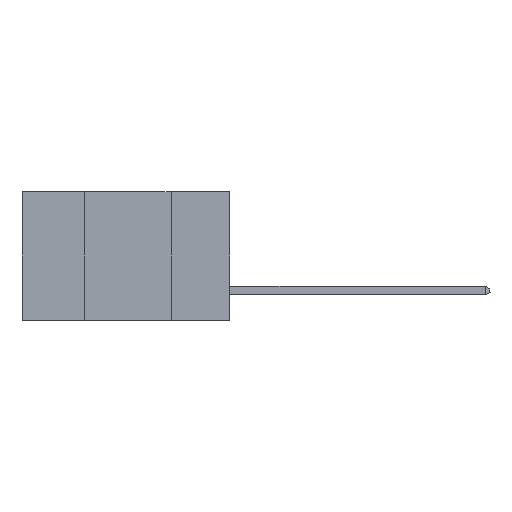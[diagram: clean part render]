
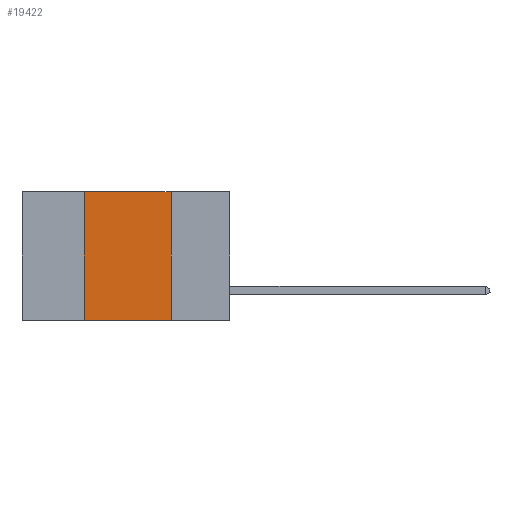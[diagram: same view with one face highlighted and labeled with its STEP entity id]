
A CAD part, left-side view. The second image highlights one B-rep face of the part: STEP entity #19422.
In plain terms, the highlighted planar face has unit normal (-1, 0, 0).
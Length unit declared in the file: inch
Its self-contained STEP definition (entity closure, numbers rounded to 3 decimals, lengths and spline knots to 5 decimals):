
#303 = DIRECTION ( 'NONE',  ( 0., 0., -1. ) ) ;
#1326 = EDGE_CURVE ( 'NONE', #4661, #2006, #3952, .T. ) ;
#1372 = EDGE_CURVE ( 'NONE', #2006, #10622, #6803, .T. ) ;
#1980 = CARTESIAN_POINT ( 'NONE',  ( 0., 0.6, -0.37 ) ) ;
#2006 = VERTEX_POINT ( 'NONE', #17295 ) ;
#2406 = AXIS2_PLACEMENT_3D ( 'NONE', #7477, #11093, #303 ) ;
#2669 = FACE_OUTER_BOUND ( 'NONE', #4055, .T. ) ;
#2973 = CARTESIAN_POINT ( 'NONE',  ( 0., 0.42, 0. ) ) ;
#3263 = VERTEX_POINT ( 'NONE', #16446 ) ;
#3813 = PLANE ( 'NONE',  #2406 ) ;
#3952 = LINE ( 'NONE', #4506, #13008 ) ;
#4055 = EDGE_LOOP ( 'NONE', ( #18045, #22132, #10063, #14865 ) ) ;
#4413 = CARTESIAN_POINT ( 'NONE',  ( 0., 0.17, -0.37 ) ) ;
#4506 = CARTESIAN_POINT ( 'NONE',  ( 0., 0.6, 0. ) ) ;
#4661 = VERTEX_POINT ( 'NONE', #17422 ) ;
#5403 = EDGE_CURVE ( 'NONE', #3263, #4661, #11404, .T. ) ;
#6803 = LINE ( 'NONE', #8231, #8215 ) ;
#7477 = CARTESIAN_POINT ( 'NONE',  ( 0., 0.6, 0. ) ) ;
#8215 = VECTOR ( 'NONE', #9796, 39.37008 ) ;
#8231 = CARTESIAN_POINT ( 'NONE',  ( 0., 0.17, 0. ) ) ;
#8276 = DIRECTION ( 'NONE',  ( 0., 0., 1. ) ) ;
#9098 = VECTOR ( 'NONE', #16268, 39.37008 ) ;
#9796 = DIRECTION ( 'NONE',  ( 0., 0., -1. ) ) ;
#10063 = ORIENTED_EDGE ( 'NONE', *, *, #5403, .F. ) ;
#10622 = VERTEX_POINT ( 'NONE', #4413 ) ;
#11093 = DIRECTION ( 'NONE',  ( 1., 0., 0. ) ) ;
#11404 = LINE ( 'NONE', #2973, #12790 ) ;
#12186 = LINE ( 'NONE', #1980, #9098 ) ;
#12790 = VECTOR ( 'NONE', #8276, 39.37008 ) ;
#13008 = VECTOR ( 'NONE', #13346, 39.37008 ) ;
#13346 = DIRECTION ( 'NONE',  ( 0., -1., 0. ) ) ;
#14865 = ORIENTED_EDGE ( 'NONE', *, *, #22148, .T. ) ;
#16268 = DIRECTION ( 'NONE',  ( 0., -1., 0. ) ) ;
#16446 = CARTESIAN_POINT ( 'NONE',  ( 0., 0.42, -0.37 ) ) ;
#17295 = CARTESIAN_POINT ( 'NONE',  ( 0., 0.17, 0. ) ) ;
#17422 = CARTESIAN_POINT ( 'NONE',  ( 0., 0.42, 0. ) ) ;
#18045 = ORIENTED_EDGE ( 'NONE', *, *, #1372, .F. ) ;
#19422 = ADVANCED_FACE ( 'NONE', ( #2669 ), #3813, .F. ) ;
#22132 = ORIENTED_EDGE ( 'NONE', *, *, #1326, .F. ) ;
#22148 = EDGE_CURVE ( 'NONE', #3263, #10622, #12186, .T. ) ;
